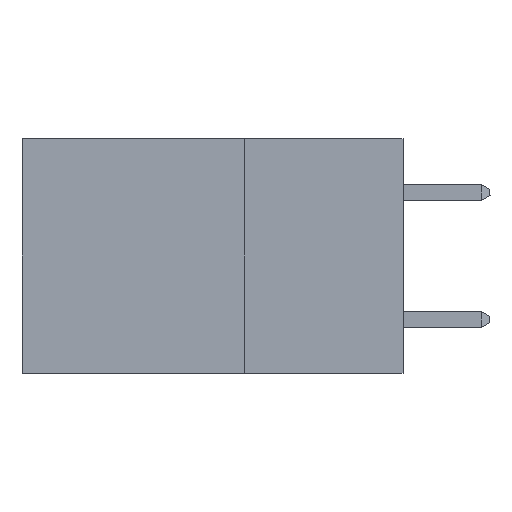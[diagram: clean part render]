
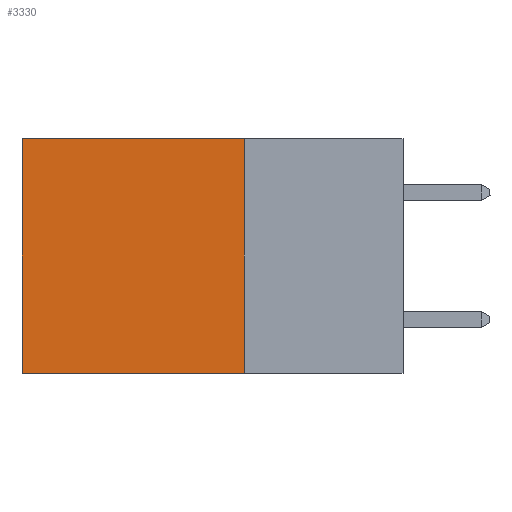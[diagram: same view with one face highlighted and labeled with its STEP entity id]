
A CAD part, left-side view. The second image highlights one B-rep face of the part: STEP entity #3330.
In plain terms, the highlighted planar face has unit normal (-1, 0, 0).
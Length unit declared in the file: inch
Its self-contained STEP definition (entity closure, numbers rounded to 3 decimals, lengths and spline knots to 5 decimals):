
#287 = VECTOR ( 'NONE', #15365, 39.37008 ) ;
#318 = EDGE_CURVE ( 'NONE', #3699, #9899, #6072, .T. ) ;
#612 = EDGE_CURVE ( 'NONE', #3610, #9899, #5593, .T. ) ;
#1869 = DIRECTION ( 'NONE',  ( 0., 0., -1. ) ) ;
#2314 = CARTESIAN_POINT ( 'NONE',  ( 0.2875, 0.25, 0. ) ) ;
#2777 = DIRECTION ( 'NONE',  ( 0., 1., 0. ) ) ;
#2876 = VECTOR ( 'NONE', #3369, 39.37008 ) ;
#3107 = VECTOR ( 'NONE', #1869, 39.37008 ) ;
#3330 = ADVANCED_FACE ( 'NONE', ( #4522 ), #11605, .F. ) ;
#3369 = DIRECTION ( 'NONE',  ( 0., 0., -1. ) ) ;
#3610 = VERTEX_POINT ( 'NONE', #12788 ) ;
#3696 = CARTESIAN_POINT ( 'NONE',  ( 0.2875, 0.6, -0.37 ) ) ;
#3699 = VERTEX_POINT ( 'NONE', #12882 ) ;
#4522 = FACE_OUTER_BOUND ( 'NONE', #9347, .T. ) ;
#5593 = LINE ( 'NONE', #5774, #5799 ) ;
#5774 = CARTESIAN_POINT ( 'NONE',  ( 0.2875, 0.25, -0.37 ) ) ;
#5799 = VECTOR ( 'NONE', #2777, 39.37008 ) ;
#5871 = AXIS2_PLACEMENT_3D ( 'NONE', #10406, #7698, #7798 ) ;
#6072 = LINE ( 'NONE', #17650, #3107 ) ;
#7307 = ORIENTED_EDGE ( 'NONE', *, *, #318, .T. ) ;
#7698 = DIRECTION ( 'NONE',  ( 1., 0., 0. ) ) ;
#7798 = DIRECTION ( 'NONE',  ( 0., 0., -1. ) ) ;
#8288 = EDGE_CURVE ( 'NONE', #8793, #3699, #12661, .T. ) ;
#8370 = ORIENTED_EDGE ( 'NONE', *, *, #612, .F. ) ;
#8793 = VERTEX_POINT ( 'NONE', #9769 ) ;
#9053 = ORIENTED_EDGE ( 'NONE', *, *, #9430, .F. ) ;
#9347 = EDGE_LOOP ( 'NONE', ( #7307, #8370, #9053, #12632 ) ) ;
#9430 = EDGE_CURVE ( 'NONE', #8793, #3610, #17383, .T. ) ;
#9704 = CARTESIAN_POINT ( 'NONE',  ( 0.2875, 0.25, 0. ) ) ;
#9769 = CARTESIAN_POINT ( 'NONE',  ( 0.2875, 0.25, 0. ) ) ;
#9899 = VERTEX_POINT ( 'NONE', #3696 ) ;
#10406 = CARTESIAN_POINT ( 'NONE',  ( 0.2875, 0.25, 0. ) ) ;
#11605 = PLANE ( 'NONE',  #5871 ) ;
#12632 = ORIENTED_EDGE ( 'NONE', *, *, #8288, .T. ) ;
#12661 = LINE ( 'NONE', #9704, #287 ) ;
#12788 = CARTESIAN_POINT ( 'NONE',  ( 0.2875, 0.25, -0.37 ) ) ;
#12882 = CARTESIAN_POINT ( 'NONE',  ( 0.2875, 0.6, 0. ) ) ;
#15365 = DIRECTION ( 'NONE',  ( 0., 1., 0. ) ) ;
#17383 = LINE ( 'NONE', #2314, #2876 ) ;
#17650 = CARTESIAN_POINT ( 'NONE',  ( 0.2875, 0.6, 0. ) ) ;
